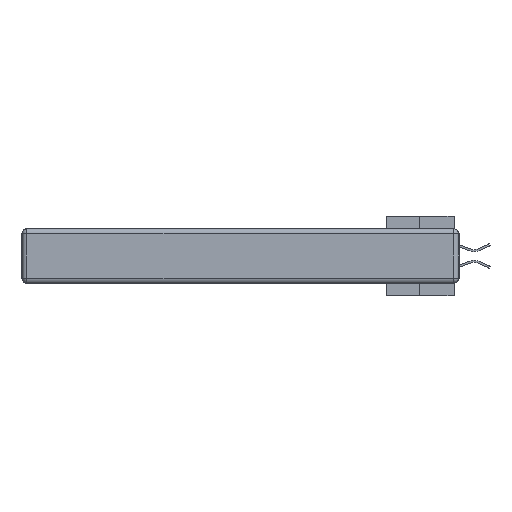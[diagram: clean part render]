
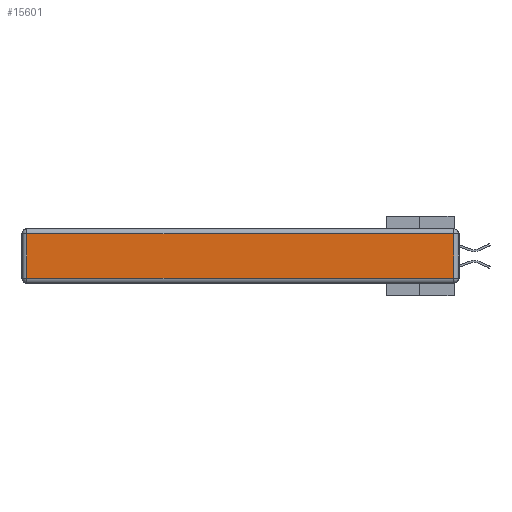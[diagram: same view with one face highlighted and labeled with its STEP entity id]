
A CAD part, left-side view. The second image highlights one B-rep face of the part: STEP entity #15601.
In plain terms, the highlighted planar face has unit normal (-1, 0, 0).
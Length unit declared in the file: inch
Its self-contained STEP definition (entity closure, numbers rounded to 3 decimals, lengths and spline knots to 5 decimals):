
#1080 = EDGE_CURVE ( 'NONE', #2829, #20333, #23170, .T. ) ;
#2829 = VERTEX_POINT ( 'NONE', #8704 ) ;
#4233 = CARTESIAN_POINT ( 'NONE',  ( 0., 2.75, -0.03 ) ) ;
#5252 = FACE_OUTER_BOUND ( 'NONE', #12795, .T. ) ;
#7007 = DIRECTION ( 'NONE',  ( 0., 0., 1. ) ) ;
#7463 = LINE ( 'NONE', #18562, #27061 ) ;
#8704 = CARTESIAN_POINT ( 'NONE',  ( 0., 0.03, -0.03 ) ) ;
#11267 = AXIS2_PLACEMENT_3D ( 'NONE', #29795, #33241, #7007 ) ;
#12795 = EDGE_LOOP ( 'NONE', ( #18589, #15248, #40383, #29751 ) ) ;
#13265 = CARTESIAN_POINT ( 'NONE',  ( 0., 2.72, -0.03 ) ) ;
#15248 = ORIENTED_EDGE ( 'NONE', *, *, #30648, .T. ) ;
#15424 = VECTOR ( 'NONE', #36493, 39.37008 ) ;
#15489 = LINE ( 'NONE', #38280, #29540 ) ;
#15601 = ADVANCED_FACE ( 'NONE', ( #5252 ), #23153, .T. ) ;
#16889 = VECTOR ( 'NONE', #36188, 39.37008 ) ;
#18562 = CARTESIAN_POINT ( 'NONE',  ( 0., 2.72, -0.343 ) ) ;
#18589 = ORIENTED_EDGE ( 'NONE', *, *, #22086, .T. ) ;
#20333 = VERTEX_POINT ( 'NONE', #13265 ) ;
#22086 = EDGE_CURVE ( 'NONE', #29383, #38004, #15489, .T. ) ;
#23153 = PLANE ( 'NONE',  #11267 ) ;
#23170 = LINE ( 'NONE', #4233, #15424 ) ;
#23322 = CARTESIAN_POINT ( 'NONE',  ( 0., 0.03, -0.313 ) ) ;
#25718 = LINE ( 'NONE', #30144, #16889 ) ;
#27061 = VECTOR ( 'NONE', #31203, 39.37008 ) ;
#29383 = VERTEX_POINT ( 'NONE', #38490 ) ;
#29540 = VECTOR ( 'NONE', #34665, 39.37008 ) ;
#29751 = ORIENTED_EDGE ( 'NONE', *, *, #33802, .T. ) ;
#29795 = CARTESIAN_POINT ( 'NONE',  ( 0., 0., -0.343 ) ) ;
#30144 = CARTESIAN_POINT ( 'NONE',  ( 0., 0.03, -0.343 ) ) ;
#30648 = EDGE_CURVE ( 'NONE', #38004, #2829, #25718, .T. ) ;
#31203 = DIRECTION ( 'NONE',  ( 0., 0., -1. ) ) ;
#33241 = DIRECTION ( 'NONE',  ( -1., 0., 0. ) ) ;
#33802 = EDGE_CURVE ( 'NONE', #20333, #29383, #7463, .T. ) ;
#34665 = DIRECTION ( 'NONE',  ( 0., -1., 0. ) ) ;
#36188 = DIRECTION ( 'NONE',  ( 0., 0., 1. ) ) ;
#36493 = DIRECTION ( 'NONE',  ( 0., 1., 0. ) ) ;
#38004 = VERTEX_POINT ( 'NONE', #23322 ) ;
#38280 = CARTESIAN_POINT ( 'NONE',  ( 0., 0., -0.313 ) ) ;
#38490 = CARTESIAN_POINT ( 'NONE',  ( 0., 2.72, -0.313 ) ) ;
#40383 = ORIENTED_EDGE ( 'NONE', *, *, #1080, .T. ) ;
